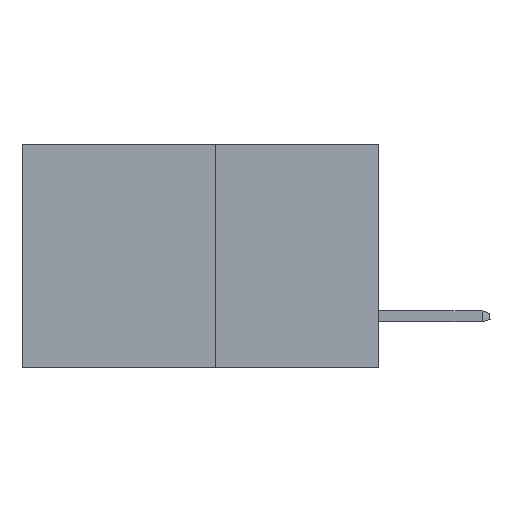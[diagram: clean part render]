
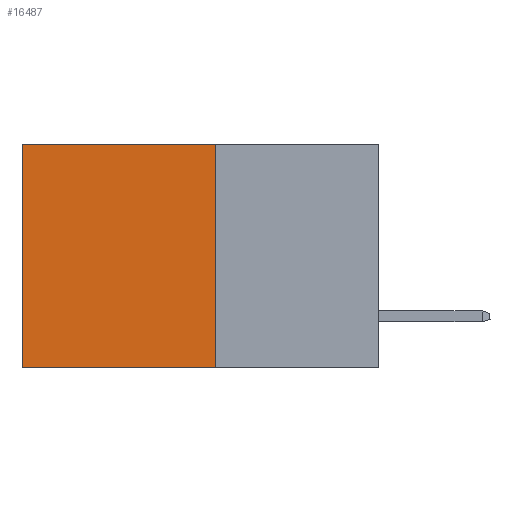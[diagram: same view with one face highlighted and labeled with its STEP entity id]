
A CAD part, left-side view. The second image highlights one B-rep face of the part: STEP entity #16487.
In plain terms, the highlighted planar face has unit normal (-1, 0, 0).
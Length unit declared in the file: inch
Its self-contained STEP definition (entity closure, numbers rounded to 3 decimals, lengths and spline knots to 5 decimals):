
#389 = VERTEX_POINT ( 'NONE', #15791 ) ;
#913 = CARTESIAN_POINT ( 'NONE',  ( 0.277, 0.27, -0.37 ) ) ;
#1611 = CARTESIAN_POINT ( 'NONE',  ( 0.277, 0.27, -0.37 ) ) ;
#2658 = CARTESIAN_POINT ( 'NONE',  ( 0.277, 0.59, 0. ) ) ;
#2865 = ORIENTED_EDGE ( 'NONE', *, *, #8621, .F. ) ;
#3838 = VECTOR ( 'NONE', #13449, 39.37008 ) ;
#5410 = VECTOR ( 'NONE', #14743, 39.37008 ) ;
#5616 = ORIENTED_EDGE ( 'NONE', *, *, #17691, .T. ) ;
#5902 = DIRECTION ( 'NONE',  ( 0., 0., -1. ) ) ;
#6338 = ORIENTED_EDGE ( 'NONE', *, *, #18442, .T. ) ;
#6884 = LINE ( 'NONE', #7901, #15905 ) ;
#7633 = VERTEX_POINT ( 'NONE', #2658 ) ;
#7825 = LINE ( 'NONE', #17803, #16327 ) ;
#7901 = CARTESIAN_POINT ( 'NONE',  ( 0.277, 0.27, -0.37 ) ) ;
#8006 = EDGE_LOOP ( 'NONE', ( #5616, #2865, #9248, #6338 ) ) ;
#8034 = CARTESIAN_POINT ( 'NONE',  ( 0.277, 0.59, -0.37 ) ) ;
#8621 = EDGE_CURVE ( 'NONE', #14711, #20371, #12854, .T. ) ;
#8777 = DIRECTION ( 'NONE',  ( 0., 0., -1. ) ) ;
#9248 = ORIENTED_EDGE ( 'NONE', *, *, #21577, .F. ) ;
#9935 = LINE ( 'NONE', #19840, #5410 ) ;
#11864 = FACE_OUTER_BOUND ( 'NONE', #8006, .T. ) ;
#12553 = AXIS2_PLACEMENT_3D ( 'NONE', #17248, #13794, #8777 ) ;
#12854 = LINE ( 'NONE', #1611, #3838 ) ;
#13015 = DIRECTION ( 'NONE',  ( 0., 0., -1. ) ) ;
#13449 = DIRECTION ( 'NONE',  ( 0., 1., 0. ) ) ;
#13794 = DIRECTION ( 'NONE',  ( 1., 0., 0. ) ) ;
#14711 = VERTEX_POINT ( 'NONE', #913 ) ;
#14743 = DIRECTION ( 'NONE',  ( 0., 1., 0. ) ) ;
#15791 = CARTESIAN_POINT ( 'NONE',  ( 0.277, 0.27, 0. ) ) ;
#15905 = VECTOR ( 'NONE', #13015, 39.37008 ) ;
#16327 = VECTOR ( 'NONE', #5902, 39.37008 ) ;
#16487 = ADVANCED_FACE ( 'NONE', ( #11864 ), #18958, .F. ) ;
#17248 = CARTESIAN_POINT ( 'NONE',  ( 0.277, 0.27, -0.37 ) ) ;
#17691 = EDGE_CURVE ( 'NONE', #7633, #20371, #7825, .T. ) ;
#17803 = CARTESIAN_POINT ( 'NONE',  ( 0.277, 0.59, -0.37 ) ) ;
#18442 = EDGE_CURVE ( 'NONE', #389, #7633, #9935, .T. ) ;
#18958 = PLANE ( 'NONE',  #12553 ) ;
#19840 = CARTESIAN_POINT ( 'NONE',  ( 0.277, 0.27, 0. ) ) ;
#20371 = VERTEX_POINT ( 'NONE', #8034 ) ;
#21577 = EDGE_CURVE ( 'NONE', #389, #14711, #6884, .T. ) ;
